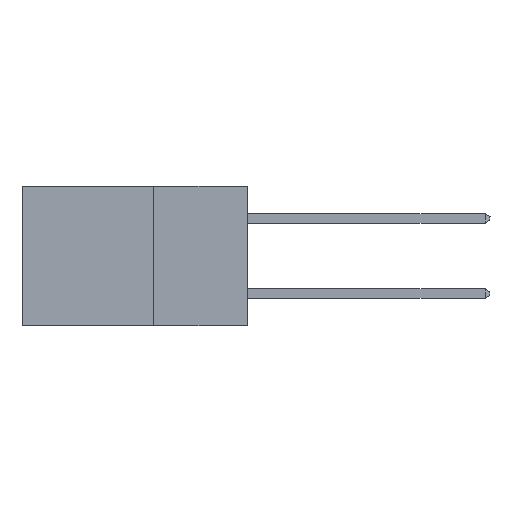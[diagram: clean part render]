
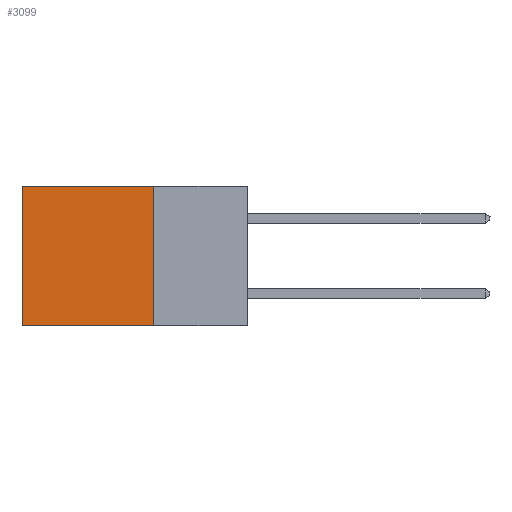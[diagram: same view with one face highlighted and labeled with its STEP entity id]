
A CAD part, left-side view. The second image highlights one B-rep face of the part: STEP entity #3099.
In plain terms, the highlighted planar face has unit normal (-1, 0, 0).
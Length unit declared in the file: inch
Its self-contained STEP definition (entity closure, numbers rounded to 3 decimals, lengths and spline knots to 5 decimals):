
#3 = CARTESIAN_POINT ( 'NONE',  ( 0.2615, 0.25, -0.37 ) ) ;
#95 = DIRECTION ( 'NONE',  ( 0., 0., -1. ) ) ;
#534 = LINE ( 'NONE', #7628, #19966 ) ;
#598 = CARTESIAN_POINT ( 'NONE',  ( 0.2615, 0.25, 0. ) ) ;
#989 = VERTEX_POINT ( 'NONE', #14711 ) ;
#2382 = EDGE_CURVE ( 'NONE', #11144, #12821, #19533, .T. ) ;
#3099 = ADVANCED_FACE ( 'NONE', ( #19303 ), #16046, .F. ) ;
#3234 = CARTESIAN_POINT ( 'NONE',  ( 0.2615, 0.25, -0.37 ) ) ;
#3582 = CARTESIAN_POINT ( 'NONE',  ( 0.2615, 0.6, -0.37 ) ) ;
#7628 = CARTESIAN_POINT ( 'NONE',  ( 0.2615, 0.25, -0.37 ) ) ;
#7655 = CARTESIAN_POINT ( 'NONE',  ( 0.2615, 0.6, -0.37 ) ) ;
#8222 = EDGE_CURVE ( 'NONE', #12821, #18880, #21843, .T. ) ;
#8689 = VECTOR ( 'NONE', #20348, 39.37008 ) ;
#8838 = DIRECTION ( 'NONE',  ( 0., 0., -1. ) ) ;
#10472 = LINE ( 'NONE', #3, #11091 ) ;
#10603 = ORIENTED_EDGE ( 'NONE', *, *, #13893, .F. ) ;
#11091 = VECTOR ( 'NONE', #8838, 39.37008 ) ;
#11144 = VERTEX_POINT ( 'NONE', #598 ) ;
#12435 = CARTESIAN_POINT ( 'NONE',  ( 0.2615, 0.25, 0. ) ) ;
#12521 = EDGE_CURVE ( 'NONE', #989, #18880, #534, .T. ) ;
#12821 = VERTEX_POINT ( 'NONE', #15660 ) ;
#12907 = AXIS2_PLACEMENT_3D ( 'NONE', #3234, #19179, #95 ) ;
#13008 = DIRECTION ( 'NONE',  ( 0., 1., 0. ) ) ;
#13136 = ORIENTED_EDGE ( 'NONE', *, *, #12521, .F. ) ;
#13893 = EDGE_CURVE ( 'NONE', #11144, #989, #10472, .T. ) ;
#14228 = ORIENTED_EDGE ( 'NONE', *, *, #8222, .T. ) ;
#14526 = DIRECTION ( 'NONE',  ( 0., 1., 0. ) ) ;
#14711 = CARTESIAN_POINT ( 'NONE',  ( 0.2615, 0.25, -0.37 ) ) ;
#15660 = CARTESIAN_POINT ( 'NONE',  ( 0.2615, 0.6, 0. ) ) ;
#16046 = PLANE ( 'NONE',  #12907 ) ;
#17091 = EDGE_LOOP ( 'NONE', ( #14228, #13136, #10603, #18146 ) ) ;
#18146 = ORIENTED_EDGE ( 'NONE', *, *, #2382, .T. ) ;
#18550 = VECTOR ( 'NONE', #14526, 39.37008 ) ;
#18880 = VERTEX_POINT ( 'NONE', #3582 ) ;
#19179 = DIRECTION ( 'NONE',  ( 1., 0., 0. ) ) ;
#19303 = FACE_OUTER_BOUND ( 'NONE', #17091, .T. ) ;
#19533 = LINE ( 'NONE', #12435, #18550 ) ;
#19966 = VECTOR ( 'NONE', #13008, 39.37008 ) ;
#20348 = DIRECTION ( 'NONE',  ( 0., 0., -1. ) ) ;
#21843 = LINE ( 'NONE', #7655, #8689 ) ;
